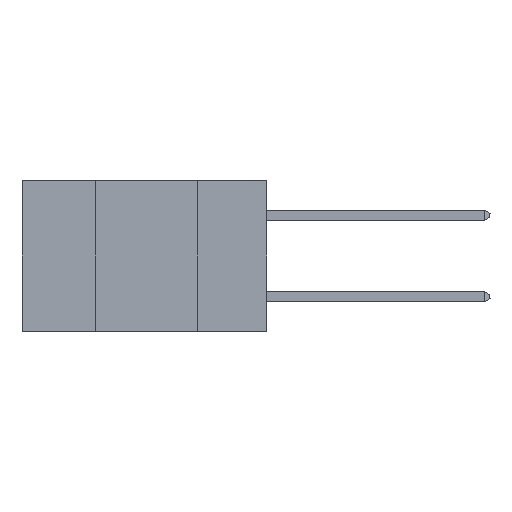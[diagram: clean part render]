
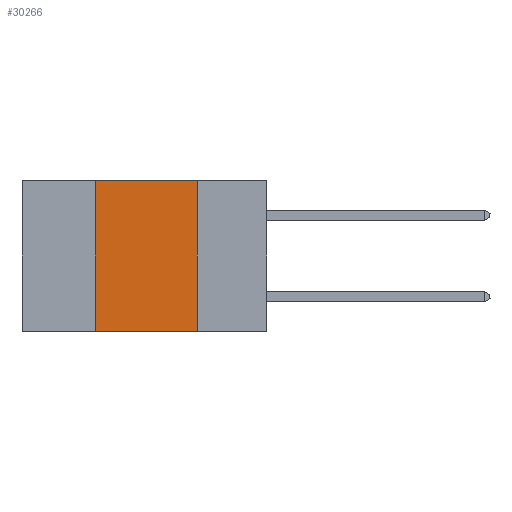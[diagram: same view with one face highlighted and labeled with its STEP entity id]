
A CAD part, left-side view. The second image highlights one B-rep face of the part: STEP entity #30266.
In plain terms, the highlighted planar face has unit normal (-1, 0, 0).
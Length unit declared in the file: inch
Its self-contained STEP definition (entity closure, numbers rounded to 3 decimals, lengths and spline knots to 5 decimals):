
#286 = ORIENTED_EDGE ( 'NONE', *, *, #2369, .F. ) ;
#565 = DIRECTION ( 'NONE',  ( 0., -1., 0. ) ) ;
#770 = CARTESIAN_POINT ( 'NONE',  ( 0., 0.17, 0. ) ) ;
#1509 = DIRECTION ( 'NONE',  ( 1., 0., 0. ) ) ;
#1741 = LINE ( 'NONE', #11524, #17468 ) ;
#1810 = EDGE_LOOP ( 'NONE', ( #4876, #286, #34761, #4611 ) ) ;
#2369 = EDGE_CURVE ( 'NONE', #12589, #26774, #38615, .T. ) ;
#2972 = VECTOR ( 'NONE', #6480, 39.37008 ) ;
#4556 = DIRECTION ( 'NONE',  ( 0., 0., -1. ) ) ;
#4611 = ORIENTED_EDGE ( 'NONE', *, *, #29889, .T. ) ;
#4876 = ORIENTED_EDGE ( 'NONE', *, *, #11634, .F. ) ;
#4958 = PLANE ( 'NONE',  #29105 ) ;
#5653 = EDGE_CURVE ( 'NONE', #12601, #12589, #35446, .T. ) ;
#6046 = DIRECTION ( 'NONE',  ( 0., -1., 0. ) ) ;
#6480 = DIRECTION ( 'NONE',  ( 0., 0., 1. ) ) ;
#11524 = CARTESIAN_POINT ( 'NONE',  ( 0., 0.6, -0.37 ) ) ;
#11634 = EDGE_CURVE ( 'NONE', #26774, #20336, #20113, .T. ) ;
#11878 = VECTOR ( 'NONE', #565, 39.37008 ) ;
#12589 = VERTEX_POINT ( 'NONE', #20958 ) ;
#12601 = VERTEX_POINT ( 'NONE', #16097 ) ;
#16097 = CARTESIAN_POINT ( 'NONE',  ( 0., 0.42, -0.37 ) ) ;
#17468 = VECTOR ( 'NONE', #6046, 39.37008 ) ;
#19920 = CARTESIAN_POINT ( 'NONE',  ( 0., 0.17, -0.37 ) ) ;
#20113 = LINE ( 'NONE', #23008, #35871 ) ;
#20336 = VERTEX_POINT ( 'NONE', #19920 ) ;
#20958 = CARTESIAN_POINT ( 'NONE',  ( 0., 0.42, 0. ) ) ;
#23008 = CARTESIAN_POINT ( 'NONE',  ( 0., 0.17, 0. ) ) ;
#26774 = VERTEX_POINT ( 'NONE', #770 ) ;
#27585 = CARTESIAN_POINT ( 'NONE',  ( 0., 0.42, 0. ) ) ;
#28055 = CARTESIAN_POINT ( 'NONE',  ( 0., 0.6, 0. ) ) ;
#28423 = FACE_OUTER_BOUND ( 'NONE', #1810, .T. ) ;
#29105 = AXIS2_PLACEMENT_3D ( 'NONE', #31776, #1509, #4556 ) ;
#29175 = DIRECTION ( 'NONE',  ( 0., 0., -1. ) ) ;
#29889 = EDGE_CURVE ( 'NONE', #12601, #20336, #1741, .T. ) ;
#30266 = ADVANCED_FACE ( 'NONE', ( #28423 ), #4958, .F. ) ;
#31776 = CARTESIAN_POINT ( 'NONE',  ( 0., 0.6, 0. ) ) ;
#34761 = ORIENTED_EDGE ( 'NONE', *, *, #5653, .F. ) ;
#35446 = LINE ( 'NONE', #27585, #2972 ) ;
#35871 = VECTOR ( 'NONE', #29175, 39.37008 ) ;
#38615 = LINE ( 'NONE', #28055, #11878 ) ;
